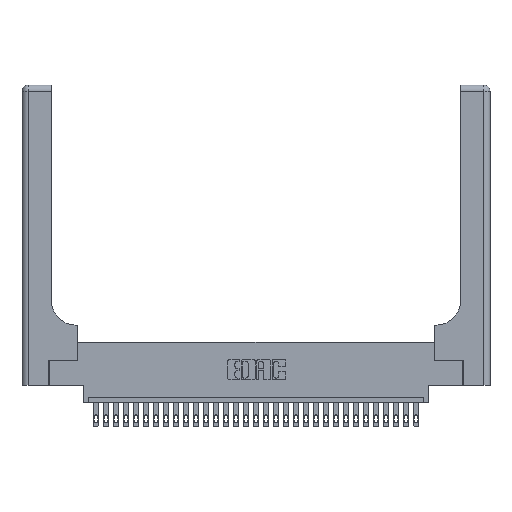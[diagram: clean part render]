
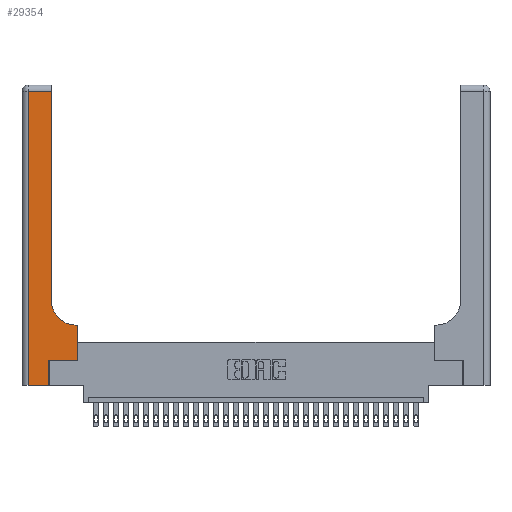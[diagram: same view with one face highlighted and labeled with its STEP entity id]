
A CAD part, top view. The second image highlights one B-rep face of the part: STEP entity #29354.
In plain terms, the highlighted planar face has unit normal (0, 0, 1).
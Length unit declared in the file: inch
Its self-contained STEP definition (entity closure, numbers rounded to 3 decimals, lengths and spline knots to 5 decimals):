
#330 = VECTOR ( 'NONE', #2659, 39.37008 ) ;
#337 = VECTOR ( 'NONE', #12394, 39.37008 ) ;
#497 = CARTESIAN_POINT ( 'NONE',  ( 0., 0., 0.37 ) ) ;
#889 = VECTOR ( 'NONE', #28452, 39.37008 ) ;
#1250 = EDGE_CURVE ( 'NONE', #16160, #8199, #2027, .T. ) ;
#1973 = VECTOR ( 'NONE', #18604, 39.37008 ) ;
#2027 = LINE ( 'NONE', #9537, #17184 ) ;
#2535 = VECTOR ( 'NONE', #14494, 39.37008 ) ;
#2659 = DIRECTION ( 'NONE',  ( 0., 1., 0. ) ) ;
#3503 = AXIS2_PLACEMENT_3D ( 'NONE', #23105, #20810, #6456 ) ;
#3576 = EDGE_CURVE ( 'NONE', #11609, #21083, #16560, .T. ) ;
#3730 = VERTEX_POINT ( 'NONE', #14196 ) ;
#4453 = LINE ( 'NONE', #7084, #29025 ) ;
#4697 = LINE ( 'NONE', #31069, #889 ) ;
#5282 = EDGE_CURVE ( 'NONE', #30876, #13335, #4697, .T. ) ;
#5438 = ORIENTED_EDGE ( 'NONE', *, *, #20712, .T. ) ;
#5952 = DIRECTION ( 'NONE',  ( 0., 0., -1. ) ) ;
#6235 = EDGE_CURVE ( 'NONE', #8199, #3730, #26873, .T. ) ;
#6360 = FACE_OUTER_BOUND ( 'NONE', #15276, .T. ) ;
#6456 = DIRECTION ( 'NONE',  ( 1., 0., 0. ) ) ;
#7084 = CARTESIAN_POINT ( 'NONE',  ( 0.06, 3., 0.37 ) ) ;
#7549 = CARTESIAN_POINT ( 'NONE',  ( 0.2915, 0.85, 0.37 ) ) ;
#8053 = VERTEX_POINT ( 'NONE', #7549 ) ;
#8060 = DIRECTION ( 'NONE',  ( 0., 1., 0. ) ) ;
#8199 = VERTEX_POINT ( 'NONE', #15415 ) ;
#8509 = PLANE ( 'NONE',  #9741 ) ;
#9114 = EDGE_CURVE ( 'NONE', #21083, #21505, #4453, .T. ) ;
#9537 = CARTESIAN_POINT ( 'NONE',  ( 0.269, 0., 0.37 ) ) ;
#9731 = ORIENTED_EDGE ( 'NONE', *, *, #5282, .T. ) ;
#9741 = AXIS2_PLACEMENT_3D ( 'NONE', #13300, #5952, #25568 ) ;
#10056 = CIRCLE ( 'NONE', #3503, 0.25 ) ;
#10066 = ORIENTED_EDGE ( 'NONE', *, *, #1250, .T. ) ;
#11609 = VERTEX_POINT ( 'NONE', #17848 ) ;
#12394 = DIRECTION ( 'NONE',  ( 1., 0., 0. ) ) ;
#13300 = CARTESIAN_POINT ( 'NONE',  ( 0., 3., 0.37 ) ) ;
#13335 = VERTEX_POINT ( 'NONE', #31208 ) ;
#13350 = ORIENTED_EDGE ( 'NONE', *, *, #22619, .T. ) ;
#14196 = CARTESIAN_POINT ( 'NONE',  ( 0.5585, 0.25, 0.37 ) ) ;
#14494 = DIRECTION ( 'NONE',  ( -1., 0., 0. ) ) ;
#14654 = ORIENTED_EDGE ( 'NONE', *, *, #6235, .T. ) ;
#15276 = EDGE_LOOP ( 'NONE', ( #16707, #25916, #25818, #24568, #10066, #14654, #5438, #9731, #13350 ) ) ;
#15415 = CARTESIAN_POINT ( 'NONE',  ( 0.269, 0.25, 0.37 ) ) ;
#15770 = CARTESIAN_POINT ( 'NONE',  ( 0.06, 0., 0.37 ) ) ;
#16160 = VERTEX_POINT ( 'NONE', #20551 ) ;
#16244 = LINE ( 'NONE', #29804, #23329 ) ;
#16275 = LINE ( 'NONE', #17070, #330 ) ;
#16560 = LINE ( 'NONE', #18197, #2535 ) ;
#16707 = ORIENTED_EDGE ( 'NONE', *, *, #20265, .T. ) ;
#16743 = CARTESIAN_POINT ( 'NONE',  ( 0.269, 0.25, 0.37 ) ) ;
#16824 = DIRECTION ( 'NONE',  ( 0., 1., 0. ) ) ;
#17070 = CARTESIAN_POINT ( 'NONE',  ( 0.2915, 3., 0.37 ) ) ;
#17184 = VECTOR ( 'NONE', #16824, 39.37008 ) ;
#17848 = CARTESIAN_POINT ( 'NONE',  ( 0.2915, 2.94, 0.37 ) ) ;
#18197 = CARTESIAN_POINT ( 'NONE',  ( 0., 2.94, 0.37 ) ) ;
#18604 = DIRECTION ( 'NONE',  ( 1., 0., 0. ) ) ;
#20265 = EDGE_CURVE ( 'NONE', #8053, #11609, #16275, .T. ) ;
#20551 = CARTESIAN_POINT ( 'NONE',  ( 0.269, 0., 0.37 ) ) ;
#20712 = EDGE_CURVE ( 'NONE', #3730, #30876, #16244, .T. ) ;
#20810 = DIRECTION ( 'NONE',  ( 0., 0., -1. ) ) ;
#21083 = VERTEX_POINT ( 'NONE', #23099 ) ;
#21112 = DIRECTION ( 'NONE',  ( 0., -1., 0. ) ) ;
#21505 = VERTEX_POINT ( 'NONE', #15770 ) ;
#22619 = EDGE_CURVE ( 'NONE', #13335, #8053, #10056, .T. ) ;
#23099 = CARTESIAN_POINT ( 'NONE',  ( 0.06, 2.94, 0.37 ) ) ;
#23105 = CARTESIAN_POINT ( 'NONE',  ( 0.5415, 0.85, 0.37 ) ) ;
#23329 = VECTOR ( 'NONE', #8060, 39.37008 ) ;
#23789 = CARTESIAN_POINT ( 'NONE',  ( 0.5585, 0.6, 0.37 ) ) ;
#24399 = EDGE_CURVE ( 'NONE', #21505, #16160, #26410, .T. ) ;
#24568 = ORIENTED_EDGE ( 'NONE', *, *, #24399, .T. ) ;
#25568 = DIRECTION ( 'NONE',  ( -1., 0., 0. ) ) ;
#25818 = ORIENTED_EDGE ( 'NONE', *, *, #9114, .T. ) ;
#25916 = ORIENTED_EDGE ( 'NONE', *, *, #3576, .T. ) ;
#26410 = LINE ( 'NONE', #497, #337 ) ;
#26873 = LINE ( 'NONE', #16743, #1973 ) ;
#28452 = DIRECTION ( 'NONE',  ( -1., 0., 0. ) ) ;
#29025 = VECTOR ( 'NONE', #21112, 39.37008 ) ;
#29354 = ADVANCED_FACE ( 'NONE', ( #6360 ), #8509, .F. ) ;
#29804 = CARTESIAN_POINT ( 'NONE',  ( 0.5585, 0.25, 0.37 ) ) ;
#30876 = VERTEX_POINT ( 'NONE', #23789 ) ;
#31069 = CARTESIAN_POINT ( 'NONE',  ( 0.2915, 0.6, 0.37 ) ) ;
#31208 = CARTESIAN_POINT ( 'NONE',  ( 0.5415, 0.6, 0.37 ) ) ;
